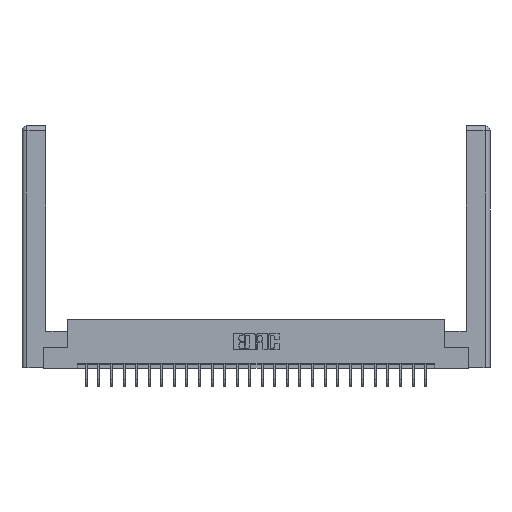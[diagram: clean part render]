
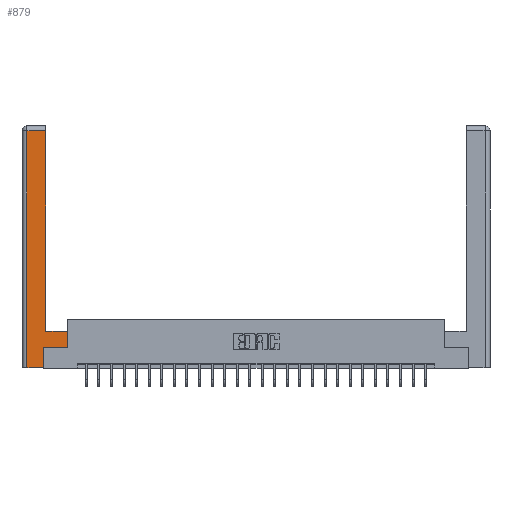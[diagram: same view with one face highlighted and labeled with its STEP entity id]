
A CAD part, top view. The second image highlights one B-rep face of the part: STEP entity #879.
In plain terms, the highlighted planar face has unit normal (0, 0, 1).
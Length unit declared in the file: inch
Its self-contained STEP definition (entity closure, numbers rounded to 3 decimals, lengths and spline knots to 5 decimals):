
#113 = LINE ( 'NONE', #23000, #15656 ) ;
#473 = DIRECTION ( 'NONE',  ( 0., 1., 0. ) ) ;
#879 = ADVANCED_FACE ( 'NONE', ( #15726 ), #17587, .F. ) ;
#1043 = CARTESIAN_POINT ( 'NONE',  ( 0.0615, 2.94, 0. ) ) ;
#1618 = LINE ( 'NONE', #13054, #18835 ) ;
#1899 = ORIENTED_EDGE ( 'NONE', *, *, #27366, .T. ) ;
#3169 = ORIENTED_EDGE ( 'NONE', *, *, #14883, .T. ) ;
#3654 = EDGE_CURVE ( 'NONE', #16815, #19041, #27362, .T. ) ;
#3655 = CARTESIAN_POINT ( 'NONE',  ( 0.265, 0.245, 0. ) ) ;
#4190 = CARTESIAN_POINT ( 'NONE',  ( 0.265, 0.245, 0. ) ) ;
#4526 = VECTOR ( 'NONE', #16961, 39.37008 ) ;
#4946 = VERTEX_POINT ( 'NONE', #1043 ) ;
#4948 = VECTOR ( 'NONE', #17745, 39.37008 ) ;
#5553 = DIRECTION ( 'NONE',  ( -1., 0., 0. ) ) ;
#5653 = VERTEX_POINT ( 'NONE', #15746 ) ;
#5749 = VECTOR ( 'NONE', #15094, 39.37008 ) ;
#6160 = VECTOR ( 'NONE', #11568, 39.37008 ) ;
#6483 = ORIENTED_EDGE ( 'NONE', *, *, #26543, .T. ) ;
#6792 = CARTESIAN_POINT ( 'NONE',  ( 0., 0., 0. ) ) ;
#6927 = ORIENTED_EDGE ( 'NONE', *, *, #3654, .T. ) ;
#7014 = EDGE_LOOP ( 'NONE', ( #26119, #1899, #6483, #8363, #3169, #24849, #6927, #21370 ) ) ;
#7193 = CARTESIAN_POINT ( 'NONE',  ( 0.0615, 0., 0. ) ) ;
#7654 = VERTEX_POINT ( 'NONE', #17734 ) ;
#7990 = CARTESIAN_POINT ( 'NONE',  ( 0.565, 0.45, 0. ) ) ;
#8329 = CARTESIAN_POINT ( 'NONE',  ( 0.565, 0.45, 0. ) ) ;
#8345 = EDGE_CURVE ( 'NONE', #22602, #7654, #24974, .T. ) ;
#8363 = ORIENTED_EDGE ( 'NONE', *, *, #18441, .T. ) ;
#10798 = CARTESIAN_POINT ( 'NONE',  ( 0.565, 0.245, 0. ) ) ;
#11525 = EDGE_CURVE ( 'NONE', #21574, #16815, #24180, .T. ) ;
#11568 = DIRECTION ( 'NONE',  ( 0., -1., 0. ) ) ;
#12878 = EDGE_CURVE ( 'NONE', #19041, #22602, #113, .T. ) ;
#13054 = CARTESIAN_POINT ( 'NONE',  ( 0.265, 0., 0. ) ) ;
#13285 = CARTESIAN_POINT ( 'NONE',  ( 0.565, 0.245, 0. ) ) ;
#13310 = DIRECTION ( 'NONE',  ( -1., 0., 0. ) ) ;
#13902 = LINE ( 'NONE', #21024, #5749 ) ;
#14883 = EDGE_CURVE ( 'NONE', #5653, #21574, #17404, .T. ) ;
#15094 = DIRECTION ( 'NONE',  ( -1., 0., 0. ) ) ;
#15207 = DIRECTION ( 'NONE',  ( 1., 0., 0. ) ) ;
#15656 = VECTOR ( 'NONE', #5553, 39.37008 ) ;
#15726 = FACE_OUTER_BOUND ( 'NONE', #7014, .T. ) ;
#15746 = CARTESIAN_POINT ( 'NONE',  ( 0.265, 0., 0. ) ) ;
#15894 = VECTOR ( 'NONE', #23143, 39.37008 ) ;
#15950 = VERTEX_POINT ( 'NONE', #21872 ) ;
#16815 = VERTEX_POINT ( 'NONE', #10798 ) ;
#16961 = DIRECTION ( 'NONE',  ( 0., 1., 0. ) ) ;
#17404 = LINE ( 'NONE', #4190, #4526 ) ;
#17587 = PLANE ( 'NONE',  #18063 ) ;
#17734 = CARTESIAN_POINT ( 'NONE',  ( 0.295, 2.94, 0. ) ) ;
#17745 = DIRECTION ( 'NONE',  ( 1., 0., 0. ) ) ;
#18063 = AXIS2_PLACEMENT_3D ( 'NONE', #6792, #21874, #13310 ) ;
#18441 = EDGE_CURVE ( 'NONE', #15950, #5653, #1618, .T. ) ;
#18835 = VECTOR ( 'NONE', #15207, 39.37008 ) ;
#19041 = VERTEX_POINT ( 'NONE', #8329 ) ;
#19251 = CARTESIAN_POINT ( 'NONE',  ( 0.295, 0.45, 0. ) ) ;
#19676 = LINE ( 'NONE', #7193, #6160 ) ;
#21024 = CARTESIAN_POINT ( 'NONE',  ( 0.0615, 2.94, 0. ) ) ;
#21370 = ORIENTED_EDGE ( 'NONE', *, *, #12878, .T. ) ;
#21574 = VERTEX_POINT ( 'NONE', #3655 ) ;
#21690 = CARTESIAN_POINT ( 'NONE',  ( 0.295, 3., 0. ) ) ;
#21872 = CARTESIAN_POINT ( 'NONE',  ( 0.0615, 0., 0. ) ) ;
#21874 = DIRECTION ( 'NONE',  ( 0., 0., -1. ) ) ;
#22602 = VERTEX_POINT ( 'NONE', #19251 ) ;
#23000 = CARTESIAN_POINT ( 'NONE',  ( 0.295, 0.45, 0. ) ) ;
#23143 = DIRECTION ( 'NONE',  ( 0., 1., 0. ) ) ;
#24180 = LINE ( 'NONE', #13285, #4948 ) ;
#24849 = ORIENTED_EDGE ( 'NONE', *, *, #11525, .T. ) ;
#24974 = LINE ( 'NONE', #21690, #25319 ) ;
#25319 = VECTOR ( 'NONE', #473, 39.37008 ) ;
#26119 = ORIENTED_EDGE ( 'NONE', *, *, #8345, .T. ) ;
#26543 = EDGE_CURVE ( 'NONE', #4946, #15950, #19676, .T. ) ;
#27362 = LINE ( 'NONE', #7990, #15894 ) ;
#27366 = EDGE_CURVE ( 'NONE', #7654, #4946, #13902, .T. ) ;
